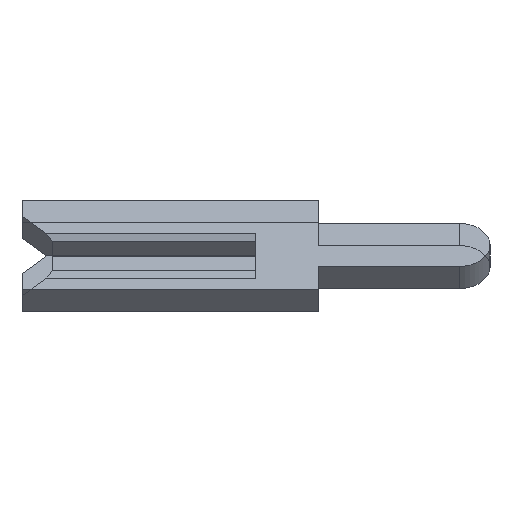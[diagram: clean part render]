
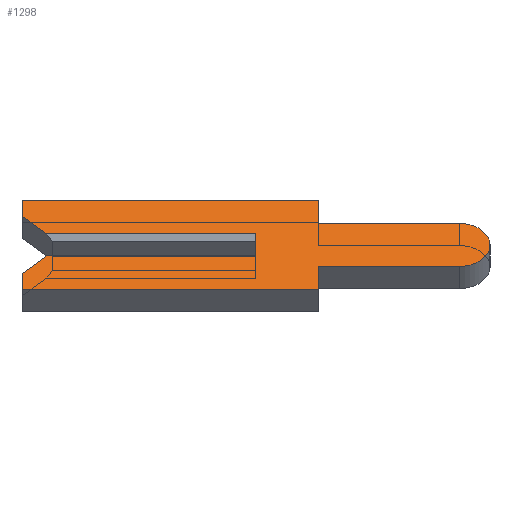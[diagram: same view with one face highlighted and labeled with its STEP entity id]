
A CAD part, left-side view. The second image highlights one B-rep face of the part: STEP entity #1298.
In plain terms, the highlighted face is planar.
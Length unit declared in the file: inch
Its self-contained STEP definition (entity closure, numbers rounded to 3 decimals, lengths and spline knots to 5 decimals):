
#27 = CARTESIAN_POINT ( 'NONE',  ( -0.01, 0.15, 0.04 ) ) ;
#34 = ORIENTED_EDGE ( 'NONE', *, *, #930, .F. ) ;
#37 = LINE ( 'NONE', #701, #1527 ) ;
#89 = DIRECTION ( 'NONE',  ( 0., -0.707, 0.707 ) ) ;
#195 = DIRECTION ( 'NONE',  ( 0., -1., 0. ) ) ;
#220 = LINE ( 'NONE', #838, #296 ) ;
#235 = ORIENTED_EDGE ( 'NONE', *, *, #898, .F. ) ;
#266 = ORIENTED_EDGE ( 'NONE', *, *, #1416, .F. ) ;
#296 = VECTOR ( 'NONE', #319, 39.37008 ) ;
#314 = CARTESIAN_POINT ( 'NONE',  ( -0.01, 0.15, -0.04 ) ) ;
#319 = DIRECTION ( 'NONE',  ( 0., -1., 0. ) ) ;
#325 = DIRECTION ( 'NONE',  ( 0., 1., 0. ) ) ;
#341 = CARTESIAN_POINT ( 'NONE',  ( -0.01, 0., -0.01 ) ) ;
#410 = LINE ( 'NONE', #1883, #640 ) ;
#419 = CARTESIAN_POINT ( 'NONE',  ( -0.01, 0.15, 0.04 ) ) ;
#422 = VERTEX_POINT ( 'NONE', #419 ) ;
#435 = LINE ( 'NONE', #1183, #2010 ) ;
#447 = VERTEX_POINT ( 'NONE', #773 ) ;
#449 = ORIENTED_EDGE ( 'NONE', *, *, #1295, .F. ) ;
#452 = EDGE_CURVE ( 'NONE', #1977, #842, #1944, .T. ) ;
#468 = DIRECTION ( 'NONE',  ( 0., 0., -1. ) ) ;
#484 = VECTOR ( 'NONE', #1010, 39.37008 ) ;
#495 = CARTESIAN_POINT ( 'NONE',  ( -0.01, 0.15, -0.026 ) ) ;
#510 = ORIENTED_EDGE ( 'NONE', *, *, #777, .T. ) ;
#511 = PLANE ( 'NONE',  #882 ) ;
#535 = CARTESIAN_POINT ( 'NONE',  ( -0.01, -0.04, -0.04 ) ) ;
#558 = ORIENTED_EDGE ( 'NONE', *, *, #1042, .F. ) ;
#562 = LINE ( 'NONE', #1037, #1874 ) ;
#574 = EDGE_CURVE ( 'NONE', #1869, #422, #410, .T. ) ;
#601 = EDGE_CURVE ( 'NONE', #1450, #1631, #562, .T. ) ;
#640 = VECTOR ( 'NONE', #1866, 39.37008 ) ;
#666 = DIRECTION ( 'NONE',  ( 1., 0., 0. ) ) ;
#683 = CARTESIAN_POINT ( 'NONE',  ( -0.01, 0., 0.01 ) ) ;
#696 = VERTEX_POINT ( 'NONE', #859 ) ;
#699 = LINE ( 'NONE', #1574, #2181 ) ;
#700 = EDGE_CURVE ( 'NONE', #447, #1501, #435, .T. ) ;
#701 = CARTESIAN_POINT ( 'NONE',  ( -0.01, 0.1305, 0.0065 ) ) ;
#710 = LINE ( 'NONE', #314, #1873 ) ;
#728 = FACE_OUTER_BOUND ( 'NONE', #1057, .T. ) ;
#738 = CARTESIAN_POINT ( 'NONE',  ( -0.01, 0.15, -0.04 ) ) ;
#745 = ORIENTED_EDGE ( 'NONE', *, *, #452, .F. ) ;
#773 = CARTESIAN_POINT ( 'NONE',  ( -0.01, -0.1305, -0.0195 ) ) ;
#777 = EDGE_CURVE ( 'NONE', #696, #1631, #220, .T. ) ;
#813 = ORIENTED_EDGE ( 'NONE', *, *, #966, .F. ) ;
#838 = CARTESIAN_POINT ( 'NONE',  ( -0.01, 0.15, 0.01 ) ) ;
#842 = VERTEX_POINT ( 'NONE', #2099 ) ;
#845 = ORIENTED_EDGE ( 'NONE', *, *, #1783, .F. ) ;
#859 = CARTESIAN_POINT ( 'NONE',  ( -0.01, 0.134, 0.01 ) ) ;
#882 = AXIS2_PLACEMENT_3D ( 'NONE', #1400, #1738, #1046 ) ;
#886 = CARTESIAN_POINT ( 'NONE',  ( -0.01, 0.15, -0.026 ) ) ;
#898 = EDGE_CURVE ( 'NONE', #1565, #2078, #1960, .T. ) ;
#912 = VECTOR ( 'NONE', #89, 39.37008 ) ;
#914 = ORIENTED_EDGE ( 'NONE', *, *, #574, .F. ) ;
#917 = CARTESIAN_POINT ( 'NONE',  ( -0.01, -0.1305, 0.0195 ) ) ;
#930 = EDGE_CURVE ( 'NONE', #422, #1864, #1872, .T. ) ;
#966 = EDGE_CURVE ( 'NONE', #696, #1869, #37, .T. ) ;
#993 = CARTESIAN_POINT ( 'NONE',  ( -0.01, -0.04, 0.04 ) ) ;
#1010 = DIRECTION ( 'NONE',  ( 0., -1., 0. ) ) ;
#1036 = VECTOR ( 'NONE', #195, 39.37008 ) ;
#1037 = CARTESIAN_POINT ( 'NONE',  ( -0.01, 0., 0.0065 ) ) ;
#1039 = CARTESIAN_POINT ( 'NONE',  ( -0.01, -0.04, 0.0195 ) ) ;
#1042 = EDGE_CURVE ( 'NONE', #1850, #2119, #710, .T. ) ;
#1046 = DIRECTION ( 'NONE',  ( 0., 0., -1. ) ) ;
#1057 = EDGE_LOOP ( 'NONE', ( #510, #1682, #449, #745, #2003, #558, #845, #1768, #266, #235, #1217, #34, #914, #813 ) ) ;
#1122 = EDGE_CURVE ( 'NONE', #1864, #1565, #2183, .T. ) ;
#1130 = CARTESIAN_POINT ( 'NONE',  ( -0.01, 0.1305, -0.0065 ) ) ;
#1183 = CARTESIAN_POINT ( 'NONE',  ( -0.01, -0.04, -0.0195 ) ) ;
#1207 = DIRECTION ( 'NONE',  ( 0., 0., -1. ) ) ;
#1210 = DIRECTION ( 'NONE',  ( 0., -1., 0. ) ) ;
#1217 = ORIENTED_EDGE ( 'NONE', *, *, #1122, .F. ) ;
#1232 = DIRECTION ( 'NONE',  ( 0., 0.707, 0.707 ) ) ;
#1263 = DIRECTION ( 'NONE',  ( 0., 0., -1. ) ) ;
#1295 = EDGE_CURVE ( 'NONE', #842, #1450, #699, .T. ) ;
#1298 = ADVANCED_FACE ( 'NONE', ( #728 ), #511, .F. ) ;
#1365 = DIRECTION ( 'NONE',  ( 0., 1., 0. ) ) ;
#1366 = EDGE_CURVE ( 'NONE', #2119, #1977, #1955, .T. ) ;
#1378 = DIRECTION ( 'NONE',  ( 0., 0., 1. ) ) ;
#1382 = DIRECTION ( 'NONE',  ( 0., 0., 1. ) ) ;
#1399 = VECTOR ( 'NONE', #468, 39.37008 ) ;
#1400 = CARTESIAN_POINT ( 'NONE',  ( -0.01, -0.1305, 0. ) ) ;
#1416 = EDGE_CURVE ( 'NONE', #2078, #447, #1847, .T. ) ;
#1440 = CARTESIAN_POINT ( 'NONE',  ( -0.01, 0.15, 0.026 ) ) ;
#1450 = VERTEX_POINT ( 'NONE', #341 ) ;
#1453 = CARTESIAN_POINT ( 'NONE',  ( -0.01, -0.04, -0.04 ) ) ;
#1499 = VECTOR ( 'NONE', #1382, 39.37008 ) ;
#1501 = VERTEX_POINT ( 'NONE', #2075 ) ;
#1527 = VECTOR ( 'NONE', #1232, 39.37008 ) ;
#1565 = VERTEX_POINT ( 'NONE', #1039 ) ;
#1574 = CARTESIAN_POINT ( 'NONE',  ( -0.01, -0.1305, -0.01 ) ) ;
#1631 = VERTEX_POINT ( 'NONE', #683 ) ;
#1682 = ORIENTED_EDGE ( 'NONE', *, *, #601, .F. ) ;
#1726 = CARTESIAN_POINT ( 'NONE',  ( -0.01, -0.1305, 0. ) ) ;
#1738 = DIRECTION ( 'NONE',  ( 1., 0., 0. ) ) ;
#1768 = ORIENTED_EDGE ( 'NONE', *, *, #700, .F. ) ;
#1783 = EDGE_CURVE ( 'NONE', #1501, #1850, #2144, .T. ) ;
#1847 = CIRCLE ( 'NONE', #1931, 0.0195 ) ;
#1850 = VERTEX_POINT ( 'NONE', #1453 ) ;
#1864 = VERTEX_POINT ( 'NONE', #2121 ) ;
#1866 = DIRECTION ( 'NONE',  ( 0., 0., 1. ) ) ;
#1869 = VERTEX_POINT ( 'NONE', #1440 ) ;
#1872 = LINE ( 'NONE', #27, #484 ) ;
#1873 = VECTOR ( 'NONE', #325, 39.37008 ) ;
#1874 = VECTOR ( 'NONE', #1378, 39.37008 ) ;
#1883 = CARTESIAN_POINT ( 'NONE',  ( -0.01, 0.15, 0.026 ) ) ;
#1921 = CARTESIAN_POINT ( 'NONE',  ( -0.01, -0.04, 0.0195 ) ) ;
#1931 = AXIS2_PLACEMENT_3D ( 'NONE', #1726, #666, #1207 ) ;
#1944 = LINE ( 'NONE', #1130, #912 ) ;
#1955 = LINE ( 'NONE', #495, #1499 ) ;
#1960 = LINE ( 'NONE', #1921, #1036 ) ;
#1977 = VERTEX_POINT ( 'NONE', #886 ) ;
#1980 = VECTOR ( 'NONE', #1263, 39.37008 ) ;
#2003 = ORIENTED_EDGE ( 'NONE', *, *, #1366, .F. ) ;
#2010 = VECTOR ( 'NONE', #1365, 39.37008 ) ;
#2075 = CARTESIAN_POINT ( 'NONE',  ( -0.01, -0.04, -0.0195 ) ) ;
#2078 = VERTEX_POINT ( 'NONE', #917 ) ;
#2099 = CARTESIAN_POINT ( 'NONE',  ( -0.01, 0.134, -0.01 ) ) ;
#2119 = VERTEX_POINT ( 'NONE', #738 ) ;
#2121 = CARTESIAN_POINT ( 'NONE',  ( -0.01, -0.04, 0.04 ) ) ;
#2144 = LINE ( 'NONE', #535, #1980 ) ;
#2181 = VECTOR ( 'NONE', #1210, 39.37008 ) ;
#2183 = LINE ( 'NONE', #993, #1399 ) ;
